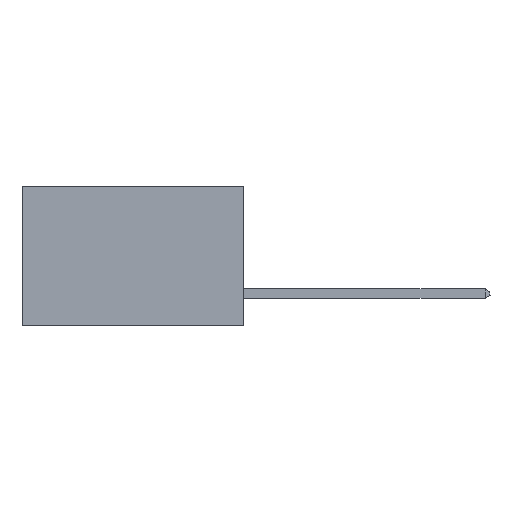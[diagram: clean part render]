
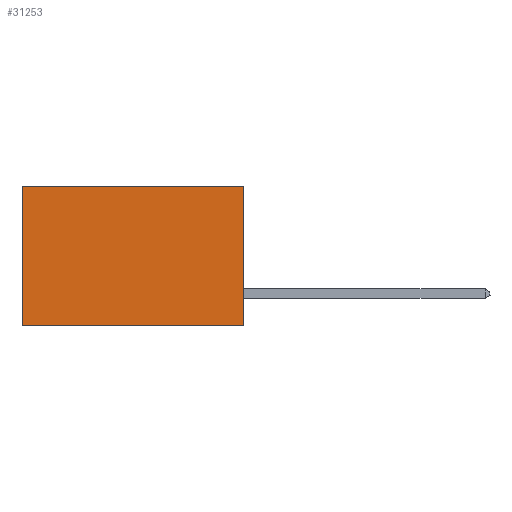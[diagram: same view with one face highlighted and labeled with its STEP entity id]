
A CAD part, left-side view. The second image highlights one B-rep face of the part: STEP entity #31253.
In plain terms, the highlighted planar face has unit normal (-1, 0, 0).
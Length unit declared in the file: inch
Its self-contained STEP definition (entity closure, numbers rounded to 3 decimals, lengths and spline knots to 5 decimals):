
#1778 = CARTESIAN_POINT ( 'NONE',  ( 0.277, 0., -0.37 ) ) ;
#1822 = VERTEX_POINT ( 'NONE', #26282 ) ;
#2135 = VERTEX_POINT ( 'NONE', #22288 ) ;
#5537 = DIRECTION ( 'NONE',  ( 0., 0., -1. ) ) ;
#5667 = EDGE_CURVE ( 'NONE', #1822, #29737, #17583, .T. ) ;
#6238 = DIRECTION ( 'NONE',  ( 0., 1., 0. ) ) ;
#6559 = ORIENTED_EDGE ( 'NONE', *, *, #16354, .T. ) ;
#6599 = DIRECTION ( 'NONE',  ( 1., 0., 0. ) ) ;
#8209 = ORIENTED_EDGE ( 'NONE', *, *, #19460, .F. ) ;
#8365 = CARTESIAN_POINT ( 'NONE',  ( 0.277, 0.59, -0.37 ) ) ;
#8736 = EDGE_CURVE ( 'NONE', #2135, #29737, #28746, .T. ) ;
#10369 = VECTOR ( 'NONE', #6238, 39.37008 ) ;
#10440 = FACE_OUTER_BOUND ( 'NONE', #27119, .T. ) ;
#10690 = ORIENTED_EDGE ( 'NONE', *, *, #8736, .T. ) ;
#11408 = CARTESIAN_POINT ( 'NONE',  ( 0.277, 0., 0. ) ) ;
#12132 = VECTOR ( 'NONE', #19360, 39.37008 ) ;
#13749 = CARTESIAN_POINT ( 'NONE',  ( 0.277, 0., 0. ) ) ;
#13783 = VERTEX_POINT ( 'NONE', #11408 ) ;
#16354 = EDGE_CURVE ( 'NONE', #13783, #2135, #16957, .T. ) ;
#16957 = LINE ( 'NONE', #13749, #10369 ) ;
#17583 = LINE ( 'NONE', #27081, #30108 ) ;
#18024 = ORIENTED_EDGE ( 'NONE', *, *, #5667, .F. ) ;
#19360 = DIRECTION ( 'NONE',  ( 0., 0., -1. ) ) ;
#19460 = EDGE_CURVE ( 'NONE', #13783, #1822, #19488, .T. ) ;
#19488 = LINE ( 'NONE', #1778, #12132 ) ;
#21488 = PLANE ( 'NONE',  #25183 ) ;
#21599 = CARTESIAN_POINT ( 'NONE',  ( 0.277, 0., -0.37 ) ) ;
#22288 = CARTESIAN_POINT ( 'NONE',  ( 0.277, 0.59, 0. ) ) ;
#24077 = DIRECTION ( 'NONE',  ( 0., 0., -1. ) ) ;
#25183 = AXIS2_PLACEMENT_3D ( 'NONE', #21599, #6599, #24077 ) ;
#26282 = CARTESIAN_POINT ( 'NONE',  ( 0.277, 0., -0.37 ) ) ;
#27081 = CARTESIAN_POINT ( 'NONE',  ( 0.277, 0., -0.37 ) ) ;
#27119 = EDGE_LOOP ( 'NONE', ( #10690, #18024, #8209, #6559 ) ) ;
#27509 = DIRECTION ( 'NONE',  ( 0., 1., 0. ) ) ;
#27955 = CARTESIAN_POINT ( 'NONE',  ( 0.277, 0.59, -0.37 ) ) ;
#27980 = VECTOR ( 'NONE', #5537, 39.37008 ) ;
#28746 = LINE ( 'NONE', #27955, #27980 ) ;
#29737 = VERTEX_POINT ( 'NONE', #8365 ) ;
#30108 = VECTOR ( 'NONE', #27509, 39.37008 ) ;
#31253 = ADVANCED_FACE ( 'NONE', ( #10440 ), #21488, .F. ) ;
